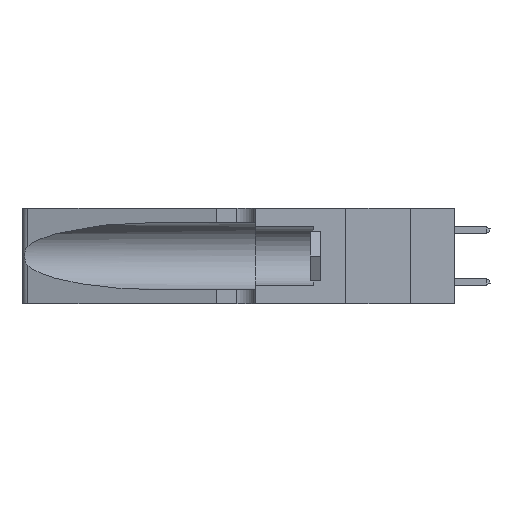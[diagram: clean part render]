
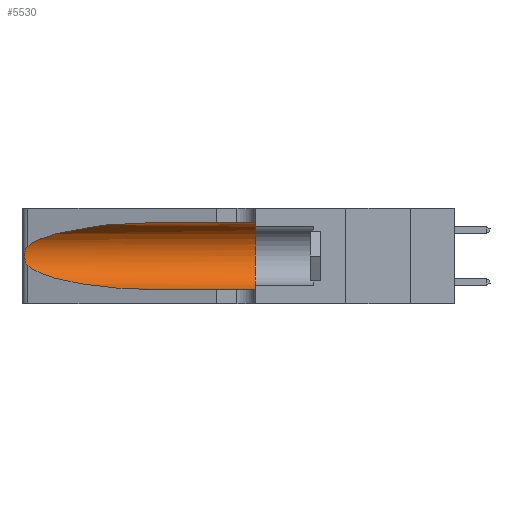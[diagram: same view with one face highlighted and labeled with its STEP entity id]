
A CAD part, left-side view. The second image highlights one B-rep face of the part: STEP entity #5530.
In plain terms, the highlighted cylindrical face has radius 3.308 mm (diameter 6.617 mm), a partial arc.
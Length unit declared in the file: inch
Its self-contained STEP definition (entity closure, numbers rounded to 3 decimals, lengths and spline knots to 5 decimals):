
#198 = CARTESIAN_POINT ( 'NONE',  ( 0.1305, 1.61858, 0.185 ) ) ;
#726 = CARTESIAN_POINT ( 'NONE',  ( 0.25487, 1.22718, 0.14631 ) ) ;
#780 = CARTESIAN_POINT ( 'NONE',  ( 0.25787, 1.23484, 0.2124 ) ) ;
#1974 = CARTESIAN_POINT ( 'NONE',  ( 0.1305, 1.61858, 0.31525 ) ) ;
#2202 = DIRECTION ( 'NONE',  ( 0., 0., -1. ) ) ;
#2690 = CARTESIAN_POINT ( 'NONE',  ( 0.18966, 0.96281, 0.31525 ) ) ;
#2745 = CARTESIAN_POINT ( 'NONE',  ( 0.26018, 1.23835, 0.19895 ) ) ;
#2983 = VERTEX_POINT ( 'NONE', #8505 ) ;
#3620 = EDGE_CURVE ( 'NONE', #14244, #2983, #13005, .T. ) ;
#3940 = CARTESIAN_POINT ( 'NONE',  ( 0.1305, 0.72297, 0.05475 ) ) ;
#4003 = VERTEX_POINT ( 'NONE', #13207 ) ;
#4697 = CARTESIAN_POINT ( 'NONE',  ( 0.26075, 1.23896, 0.178 ) ) ;
#4768 = VECTOR ( 'NONE', #7147, 39.37008 ) ;
#4822 = CARTESIAN_POINT ( 'NONE',  ( 0.18966, 0.96281, 0.05475 ) ) ;
#4974 = B_SPLINE_CURVE_WITH_KNOTS ( 'NONE', 3,
 ( #23113, #10269, #12136, #780, #13978, #2745, #15861, #4697, #17708, #6641, #19533, #8520, #21382, #10353 ),
 .UNSPECIFIED., .F., .F.,
 ( 4, 2, 2, 2, 2, 2, 4 ),
 ( 0., 0.00027, 0.00053, 0.00107, 0.0016, 0.00187, 0.00214 ),
 .UNSPECIFIED. ) ;
#5530 = ADVANCED_FACE ( 'NONE', ( #11556 ), #20768, .F. ) ;
#5757 = EDGE_LOOP ( 'NONE', ( #18822, #14330, #17713, #11138, #16750, #9462 ) ) ;
#6583 = CARTESIAN_POINT ( 'NONE',  ( 0.2373, 1.15595, 0.28018 ) ) ;
#6641 = CARTESIAN_POINT ( 'NONE',  ( 0.25856, 1.23593, 0.16098 ) ) ;
#7042 = VECTOR ( 'NONE', #20578, 39.37008 ) ;
#7147 = DIRECTION ( 'NONE',  ( 0., -1., 0. ) ) ;
#8505 = CARTESIAN_POINT ( 'NONE',  ( 0.25487, 1.22718, 0.22369 ) ) ;
#8520 = CARTESIAN_POINT ( 'NONE',  ( 0.25639, 1.23186, 0.15144 ) ) ;
#9462 = ORIENTED_EDGE ( 'NONE', *, *, #23317, .F. ) ;
#9752 = AXIS2_PLACEMENT_3D ( 'NONE', #11340, #24192, #13209 ) ;
#10269 = CARTESIAN_POINT ( 'NONE',  ( 0.25555, 1.22994, 0.2215 ) ) ;
#10353 = CARTESIAN_POINT ( 'NONE',  ( 0.25487, 1.22718, 0.14631 ) ) ;
#10634 = EDGE_CURVE ( 'NONE', #16087, #22326, #15156, .T. ) ;
#11138 = ORIENTED_EDGE ( 'NONE', *, *, #20252, .T. ) ;
#11340 = CARTESIAN_POINT ( 'NONE',  ( 0.1305, 0.35, 0.185 ) ) ;
#11556 = FACE_OUTER_BOUND ( 'NONE', #5757, .T. ) ;
#12136 = CARTESIAN_POINT ( 'NONE',  ( 0.25639, 1.23184, 0.21858 ) ) ;
#12288 = AXIS2_PLACEMENT_3D ( 'NONE', #198, #13479, #2202 ) ;
#12574 = CARTESIAN_POINT ( 'NONE',  ( 0.1305, 0.72297, 0.31525 ) ) ;
#12646 = CARTESIAN_POINT ( 'NONE',  ( 0.1305, 1.61858, 0.05475 ) ) ;
#13005 =( BOUNDED_CURVE ( )  B_SPLINE_CURVE ( 3, ( #15824, #2690, #6583, #19494 ),
 .UNSPECIFIED., .F., .T. ) 
 B_SPLINE_CURVE_WITH_KNOTS ( ( 4, 4 ),
 ( 1.5708, 2.84003 ),
 .UNSPECIFIED. ) 
 CURVE ( )  GEOMETRIC_REPRESENTATION_ITEM ( )  RATIONAL_B_SPLINE_CURVE ( ( 1., 0.87, 0.87, 1. ) ) 
 REPRESENTATION_ITEM ( '' )  );
#13207 = CARTESIAN_POINT ( 'NONE',  ( 0.1305, 0.35, 0.31525 ) ) ;
#13209 = DIRECTION ( 'NONE',  ( 0., 0., 1. ) ) ;
#13479 = DIRECTION ( 'NONE',  ( 0., -1., 0. ) ) ;
#13978 = CARTESIAN_POINT ( 'NONE',  ( 0.25854, 1.2359, 0.20912 ) ) ;
#14244 = VERTEX_POINT ( 'NONE', #12574 ) ;
#14330 = ORIENTED_EDGE ( 'NONE', *, *, #19312, .T. ) ;
#14472 = EDGE_CURVE ( 'NONE', #4003, #14959, #21946, .T. ) ;
#14959 = VERTEX_POINT ( 'NONE', #16493 ) ;
#15156 =( BOUNDED_CURVE ( )  B_SPLINE_CURVE ( 3, ( #21502, #17824, #4822, #23310 ),
 .UNSPECIFIED., .F., .T. ) 
 B_SPLINE_CURVE_WITH_KNOTS ( ( 4, 4 ),
 ( 3.44316, 4.71239 ),
 .UNSPECIFIED. ) 
 CURVE ( )  GEOMETRIC_REPRESENTATION_ITEM ( )  RATIONAL_B_SPLINE_CURVE ( ( 1., 0.87, 0.87, 1. ) ) 
 REPRESENTATION_ITEM ( '' )  );
#15824 = CARTESIAN_POINT ( 'NONE',  ( 0.1305, 0.72297, 0.31525 ) ) ;
#15861 = CARTESIAN_POINT ( 'NONE',  ( 0.26075, 1.23896, 0.19203 ) ) ;
#16087 = VERTEX_POINT ( 'NONE', #726 ) ;
#16493 = CARTESIAN_POINT ( 'NONE',  ( 0.1305, 0.35, 0.05475 ) ) ;
#16750 = ORIENTED_EDGE ( 'NONE', *, *, #14472, .F. ) ;
#17708 = CARTESIAN_POINT ( 'NONE',  ( 0.26017, 1.23833, 0.17102 ) ) ;
#17713 = ORIENTED_EDGE ( 'NONE', *, *, #10634, .T. ) ;
#17824 = CARTESIAN_POINT ( 'NONE',  ( 0.2373, 1.15595, 0.08982 ) ) ;
#18822 = ORIENTED_EDGE ( 'NONE', *, *, #3620, .T. ) ;
#19312 = EDGE_CURVE ( 'NONE', #2983, #16087, #4974, .T. ) ;
#19494 = CARTESIAN_POINT ( 'NONE',  ( 0.25487, 1.22718, 0.22369 ) ) ;
#19533 = CARTESIAN_POINT ( 'NONE',  ( 0.25789, 1.23486, 0.15765 ) ) ;
#19563 = LINE ( 'NONE', #12646, #4768 ) ;
#20252 = EDGE_CURVE ( 'NONE', #22326, #14959, #19563, .T. ) ;
#20578 = DIRECTION ( 'NONE',  ( 0., -1., 0. ) ) ;
#20768 = CYLINDRICAL_SURFACE ( 'NONE', #12288, 0.13025 ) ;
#21382 = CARTESIAN_POINT ( 'NONE',  ( 0.25555, 1.22993, 0.14849 ) ) ;
#21502 = CARTESIAN_POINT ( 'NONE',  ( 0.25487, 1.22718, 0.14631 ) ) ;
#21732 = LINE ( 'NONE', #1974, #7042 ) ;
#21946 = CIRCLE ( 'NONE', #9752, 0.13025 ) ;
#22326 = VERTEX_POINT ( 'NONE', #3940 ) ;
#23113 = CARTESIAN_POINT ( 'NONE',  ( 0.25487, 1.22718, 0.22369 ) ) ;
#23310 = CARTESIAN_POINT ( 'NONE',  ( 0.1305, 0.72297, 0.05475 ) ) ;
#23317 = EDGE_CURVE ( 'NONE', #14244, #4003, #21732, .T. ) ;
#24192 = DIRECTION ( 'NONE',  ( 0., 1., 0. ) ) ;
